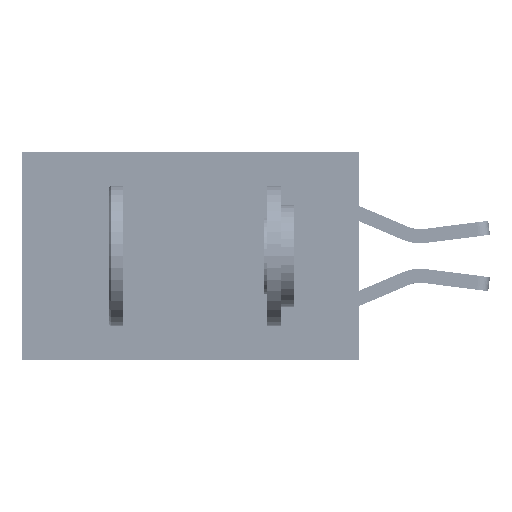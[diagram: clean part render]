
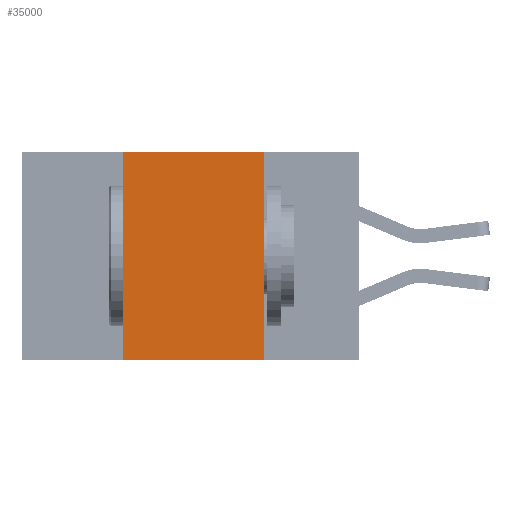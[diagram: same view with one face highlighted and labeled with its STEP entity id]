
A CAD part, left-side view. The second image highlights one B-rep face of the part: STEP entity #35000.
In plain terms, the highlighted planar face has unit normal (-1, 0, 0).
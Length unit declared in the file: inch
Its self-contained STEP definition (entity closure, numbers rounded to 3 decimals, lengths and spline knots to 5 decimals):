
#36 = EDGE_CURVE ( 'NONE', #14048, #20513, #8012, .T. ) ;
#330 = EDGE_CURVE ( 'NONE', #26364, #39974, #33466, .T. ) ;
#531 = CARTESIAN_POINT ( 'NONE',  ( 0., 0.42, -0.37 ) ) ;
#1076 = ORIENTED_EDGE ( 'NONE', *, *, #27835, .T. ) ;
#1675 = CARTESIAN_POINT ( 'NONE',  ( 0., 0.17, -0.37 ) ) ;
#3496 = DIRECTION ( 'NONE',  ( 0., 0., 1. ) ) ;
#3719 = LINE ( 'NONE', #32179, #15673 ) ;
#6549 = CARTESIAN_POINT ( 'NONE',  ( 0., 0.17, 0. ) ) ;
#7254 = AXIS2_PLACEMENT_3D ( 'NONE', #12833, #18941, #18813 ) ;
#7730 = LINE ( 'NONE', #10528, #27704 ) ;
#8012 = LINE ( 'NONE', #25122, #34499 ) ;
#9179 = ORIENTED_EDGE ( 'NONE', *, *, #36, .F. ) ;
#10048 = ORIENTED_EDGE ( 'NONE', *, *, #37516, .F. ) ;
#10528 = CARTESIAN_POINT ( 'NONE',  ( 0., 0.6, 0. ) ) ;
#12833 = CARTESIAN_POINT ( 'NONE',  ( 0., 0.6, 0. ) ) ;
#13104 = DIRECTION ( 'NONE',  ( 0., 0., -1. ) ) ;
#14048 = VERTEX_POINT ( 'NONE', #531 ) ;
#15673 = VECTOR ( 'NONE', #33005, 39.37008 ) ;
#18813 = DIRECTION ( 'NONE',  ( 0., 0., -1. ) ) ;
#18941 = DIRECTION ( 'NONE',  ( 1., 0., 0. ) ) ;
#19449 = VECTOR ( 'NONE', #13104, 39.37008 ) ;
#20513 = VERTEX_POINT ( 'NONE', #24490 ) ;
#24490 = CARTESIAN_POINT ( 'NONE',  ( 0., 0.42, 0. ) ) ;
#25122 = CARTESIAN_POINT ( 'NONE',  ( 0., 0.42, 0. ) ) ;
#25381 = PLANE ( 'NONE',  #7254 ) ;
#26364 = VERTEX_POINT ( 'NONE', #40217 ) ;
#27704 = VECTOR ( 'NONE', #32878, 39.37008 ) ;
#27835 = EDGE_CURVE ( 'NONE', #14048, #39974, #3719, .T. ) ;
#28847 = EDGE_LOOP ( 'NONE', ( #33327, #10048, #9179, #1076 ) ) ;
#32179 = CARTESIAN_POINT ( 'NONE',  ( 0., 0.6, -0.37 ) ) ;
#32878 = DIRECTION ( 'NONE',  ( 0., -1., 0. ) ) ;
#33005 = DIRECTION ( 'NONE',  ( 0., -1., 0. ) ) ;
#33218 = FACE_OUTER_BOUND ( 'NONE', #28847, .T. ) ;
#33327 = ORIENTED_EDGE ( 'NONE', *, *, #330, .F. ) ;
#33466 = LINE ( 'NONE', #6549, #19449 ) ;
#34499 = VECTOR ( 'NONE', #3496, 39.37008 ) ;
#35000 = ADVANCED_FACE ( 'NONE', ( #33218 ), #25381, .F. ) ;
#37516 = EDGE_CURVE ( 'NONE', #20513, #26364, #7730, .T. ) ;
#39974 = VERTEX_POINT ( 'NONE', #1675 ) ;
#40217 = CARTESIAN_POINT ( 'NONE',  ( 0., 0.17, 0. ) ) ;
